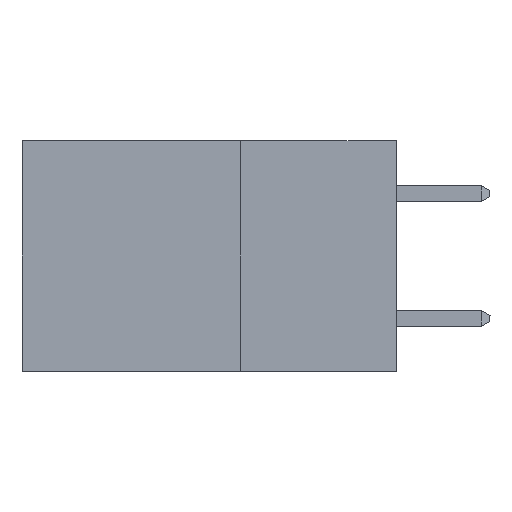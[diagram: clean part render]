
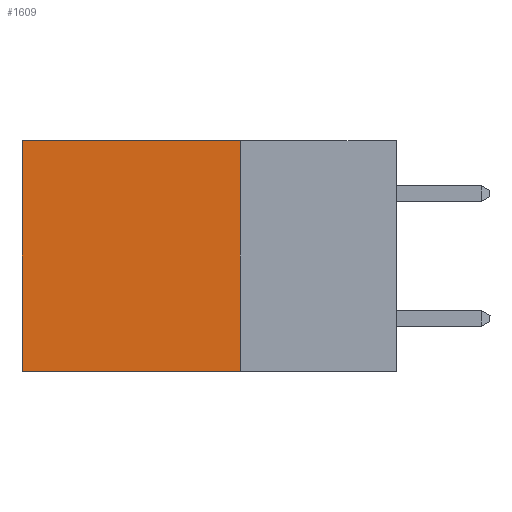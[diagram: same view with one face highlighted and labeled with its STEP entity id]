
A CAD part, left-side view. The second image highlights one B-rep face of the part: STEP entity #1609.
In plain terms, the highlighted planar face has unit normal (-1, 0, 0).
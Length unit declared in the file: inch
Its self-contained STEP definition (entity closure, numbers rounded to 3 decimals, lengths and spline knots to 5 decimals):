
#190 = DIRECTION ( 'NONE',  ( 0., 0., -1. ) ) ;
#433 = AXIS2_PLACEMENT_3D ( 'NONE', #14741, #9393, #190 ) ;
#708 = DIRECTION ( 'NONE',  ( 0., 0., -1. ) ) ;
#1050 = CARTESIAN_POINT ( 'NONE',  ( 0.298, 0.6, 0. ) ) ;
#1609 = ADVANCED_FACE ( 'NONE', ( #10508 ), #14914, .F. ) ;
#1649 = VERTEX_POINT ( 'NONE', #16003 ) ;
#1778 = VECTOR ( 'NONE', #15762, 39.37008 ) ;
#2349 = LINE ( 'NONE', #1050, #12439 ) ;
#3638 = VECTOR ( 'NONE', #8064, 39.37008 ) ;
#3689 = DIRECTION ( 'NONE',  ( 0., 0., -1. ) ) ;
#4815 = EDGE_CURVE ( 'NONE', #8227, #1649, #6329, .T. ) ;
#4981 = ORIENTED_EDGE ( 'NONE', *, *, #9461, .F. ) ;
#4984 = VERTEX_POINT ( 'NONE', #11134 ) ;
#6329 = LINE ( 'NONE', #12005, #3638 ) ;
#6774 = LINE ( 'NONE', #15198, #14643 ) ;
#7883 = ORIENTED_EDGE ( 'NONE', *, *, #4815, .T. ) ;
#8064 = DIRECTION ( 'NONE',  ( 0., 1., 0. ) ) ;
#8227 = VERTEX_POINT ( 'NONE', #9308 ) ;
#9308 = CARTESIAN_POINT ( 'NONE',  ( 0.298, 0.25, 0. ) ) ;
#9333 = VERTEX_POINT ( 'NONE', #15888 ) ;
#9393 = DIRECTION ( 'NONE',  ( 1., 0., 0. ) ) ;
#9461 = EDGE_CURVE ( 'NONE', #4984, #9333, #10446, .T. ) ;
#10446 = LINE ( 'NONE', #15867, #1778 ) ;
#10508 = FACE_OUTER_BOUND ( 'NONE', #16140, .T. ) ;
#10806 = EDGE_CURVE ( 'NONE', #8227, #4984, #6774, .T. ) ;
#11134 = CARTESIAN_POINT ( 'NONE',  ( 0.298, 0.25, -0.37 ) ) ;
#12005 = CARTESIAN_POINT ( 'NONE',  ( 0.298, 0.25, 0. ) ) ;
#12439 = VECTOR ( 'NONE', #3689, 39.37008 ) ;
#12773 = ORIENTED_EDGE ( 'NONE', *, *, #13106, .T. ) ;
#13106 = EDGE_CURVE ( 'NONE', #1649, #9333, #2349, .T. ) ;
#14243 = ORIENTED_EDGE ( 'NONE', *, *, #10806, .F. ) ;
#14643 = VECTOR ( 'NONE', #708, 39.37008 ) ;
#14741 = CARTESIAN_POINT ( 'NONE',  ( 0.298, 0.25, 0. ) ) ;
#14914 = PLANE ( 'NONE',  #433 ) ;
#15198 = CARTESIAN_POINT ( 'NONE',  ( 0.298, 0.25, 0. ) ) ;
#15762 = DIRECTION ( 'NONE',  ( 0., 1., 0. ) ) ;
#15867 = CARTESIAN_POINT ( 'NONE',  ( 0.298, 0.25, -0.37 ) ) ;
#15888 = CARTESIAN_POINT ( 'NONE',  ( 0.298, 0.6, -0.37 ) ) ;
#16003 = CARTESIAN_POINT ( 'NONE',  ( 0.298, 0.6, 0. ) ) ;
#16140 = EDGE_LOOP ( 'NONE', ( #12773, #4981, #14243, #7883 ) ) ;
